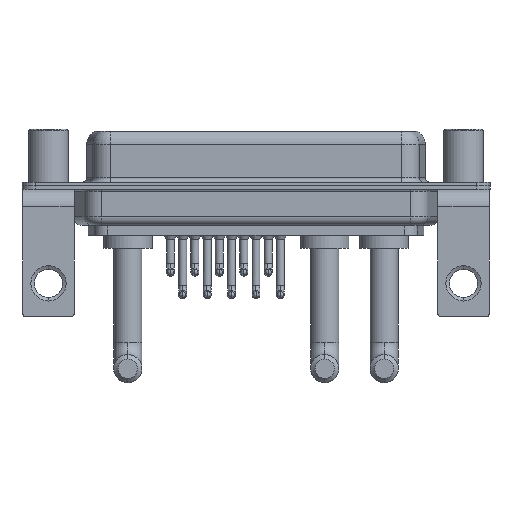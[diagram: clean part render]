
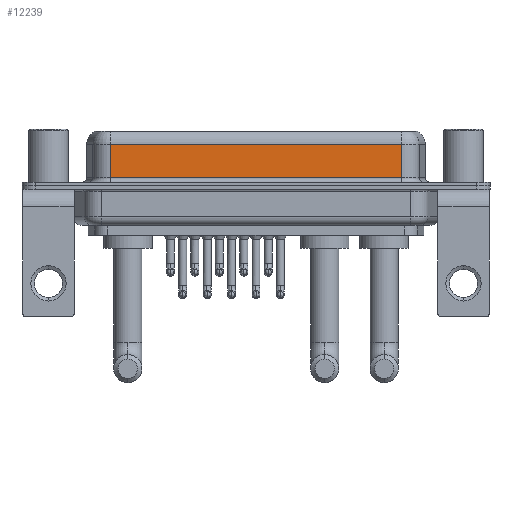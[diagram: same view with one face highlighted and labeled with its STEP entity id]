
A CAD part, front view. The second image highlights one B-rep face of the part: STEP entity #12239.
In plain terms, the highlighted planar face has unit normal (0, -1, 0).
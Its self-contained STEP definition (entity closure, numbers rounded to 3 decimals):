
#158 = EDGE_CURVE ( 'NONE', #7817, #4219, #17856, .T. ) ;
#1106 = CARTESIAN_POINT ( 'NONE',  ( 40.037, -3.95, 0.9 ) ) ;
#2630 = LINE ( 'NONE', #1106, #9734 ) ;
#2769 = CARTESIAN_POINT ( 'NONE',  ( 40.037, -3.95, 0.9 ) ) ;
#2806 = ORIENTED_EDGE ( 'NONE', *, *, #19623, .T. ) ;
#2967 = DIRECTION ( 'NONE',  ( -1., 0., 0. ) ) ;
#3245 = ORIENTED_EDGE ( 'NONE', *, *, #17838, .F. ) ;
#3484 = CARTESIAN_POINT ( 'NONE',  ( 7.013, -3.95, 0.9 ) ) ;
#3976 = PLANE ( 'NONE',  #14187 ) ;
#4219 = VERTEX_POINT ( 'NONE', #3484 ) ;
#4923 = LINE ( 'NONE', #17896, #7362 ) ;
#6803 = CARTESIAN_POINT ( 'NONE',  ( 7.013, -3.95, 6.4 ) ) ;
#7313 = LINE ( 'NONE', #9068, #15383 ) ;
#7362 = VECTOR ( 'NONE', #2967, 1000. ) ;
#7817 = VERTEX_POINT ( 'NONE', #9715 ) ;
#8222 = DIRECTION ( 'NONE',  ( 0., 0., -1. ) ) ;
#9068 = CARTESIAN_POINT ( 'NONE',  ( 40.037, -3.95, 6.4 ) ) ;
#9715 = CARTESIAN_POINT ( 'NONE',  ( 7.013, -3.95, 4.65 ) ) ;
#9734 = VECTOR ( 'NONE', #15935, 1000. ) ;
#10073 = CARTESIAN_POINT ( 'NONE',  ( 40.037, -3.95, 4.65 ) ) ;
#10405 = FACE_OUTER_BOUND ( 'NONE', #10692, .T. ) ;
#10517 = DIRECTION ( 'NONE',  ( 0., 1., 0. ) ) ;
#10557 = VERTEX_POINT ( 'NONE', #2769 ) ;
#10692 = EDGE_LOOP ( 'NONE', ( #3245, #2806, #14392, #11662 ) ) ;
#11662 = ORIENTED_EDGE ( 'NONE', *, *, #16535, .T. ) ;
#12239 = ADVANCED_FACE ( 'NONE', ( #10405 ), #3976, .F. ) ;
#13691 = CARTESIAN_POINT ( 'NONE',  ( 40.037, -3.95, 6.4 ) ) ;
#14098 = DIRECTION ( 'NONE',  ( 0., 0., -1. ) ) ;
#14187 = AXIS2_PLACEMENT_3D ( 'NONE', #13691, #10517, #15535 ) ;
#14392 = ORIENTED_EDGE ( 'NONE', *, *, #158, .T. ) ;
#15383 = VECTOR ( 'NONE', #14098, 1000. ) ;
#15535 = DIRECTION ( 'NONE',  ( 0., 0., 1. ) ) ;
#15584 = VECTOR ( 'NONE', #8222, 1000. ) ;
#15935 = DIRECTION ( 'NONE',  ( 1., 0., 0. ) ) ;
#16535 = EDGE_CURVE ( 'NONE', #4219, #10557, #2630, .T. ) ;
#17838 = EDGE_CURVE ( 'NONE', #19307, #10557, #7313, .T. ) ;
#17856 = LINE ( 'NONE', #6803, #15584 ) ;
#17896 = CARTESIAN_POINT ( 'NONE',  ( 40.037, -3.95, 4.65 ) ) ;
#19307 = VERTEX_POINT ( 'NONE', #10073 ) ;
#19623 = EDGE_CURVE ( 'NONE', #19307, #7817, #4923, .T. ) ;
